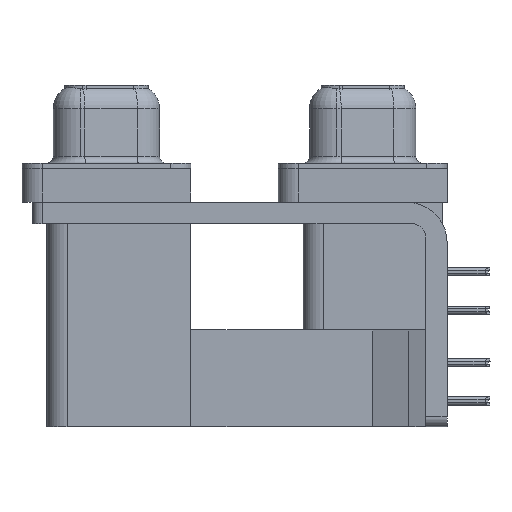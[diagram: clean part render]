
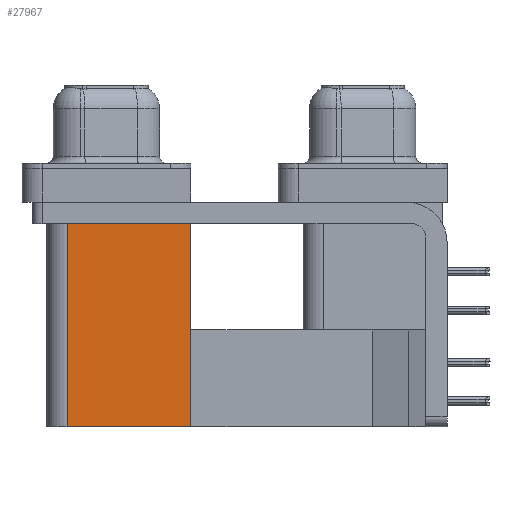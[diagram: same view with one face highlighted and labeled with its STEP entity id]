
A CAD part, left-side view. The second image highlights one B-rep face of the part: STEP entity #27967.
In plain terms, the highlighted planar face has unit normal (-1, 0, 0).
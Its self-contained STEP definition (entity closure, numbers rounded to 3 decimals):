
#82 = CARTESIAN_POINT ( 'NONE',  ( 3.79, 12.775, -19.2 ) ) ;
#305 = LINE ( 'NONE', #22608, #19377 ) ;
#399 = EDGE_CURVE ( 'NONE', #24945, #8483, #24794, .T. ) ;
#3603 = VECTOR ( 'NONE', #15435, 1000. ) ;
#3706 = EDGE_CURVE ( 'NONE', #8483, #28441, #305, .T. ) ;
#7196 = ORIENTED_EDGE ( 'NONE', *, *, #399, .T. ) ;
#8483 = VERTEX_POINT ( 'NONE', #15745 ) ;
#8659 = CARTESIAN_POINT ( 'NONE',  ( 3.79, 12.775, -19.2 ) ) ;
#10541 = CARTESIAN_POINT ( 'NONE',  ( 3.79, 12.775, -19.2 ) ) ;
#11848 = CARTESIAN_POINT ( 'NONE',  ( 3.79, 21.975, -19.2 ) ) ;
#11885 = DIRECTION ( 'NONE',  ( 0., 1., 0. ) ) ;
#13657 = VECTOR ( 'NONE', #25687, 1000. ) ;
#15435 = DIRECTION ( 'NONE',  ( 0., 0., 1. ) ) ;
#15745 = CARTESIAN_POINT ( 'NONE',  ( 3.79, 12.775, -2.5 ) ) ;
#16139 = CARTESIAN_POINT ( 'NONE',  ( 3.79, 21.975, -19.2 ) ) ;
#17267 = EDGE_LOOP ( 'NONE', ( #40820, #27397, #29177, #7196 ) ) ;
#19377 = VECTOR ( 'NONE', #35562, 1000. ) ;
#21002 = CARTESIAN_POINT ( 'NONE',  ( 3.79, 12.775, -19.2 ) ) ;
#22608 = CARTESIAN_POINT ( 'NONE',  ( 3.79, 12.775, -2.5 ) ) ;
#22734 = LINE ( 'NONE', #16139, #13657 ) ;
#23825 = VECTOR ( 'NONE', #11885, 1000. ) ;
#24794 = LINE ( 'NONE', #8659, #3603 ) ;
#24945 = VERTEX_POINT ( 'NONE', #10541 ) ;
#25687 = DIRECTION ( 'NONE',  ( 0., 0., 1. ) ) ;
#26436 = VERTEX_POINT ( 'NONE', #11848 ) ;
#27397 = ORIENTED_EDGE ( 'NONE', *, *, #31486, .F. ) ;
#27967 = ADVANCED_FACE ( 'NONE', ( #28760 ), #32171, .F. ) ;
#28006 = LINE ( 'NONE', #21002, #23825 ) ;
#28441 = VERTEX_POINT ( 'NONE', #35146 ) ;
#28760 = FACE_OUTER_BOUND ( 'NONE', #17267, .T. ) ;
#29177 = ORIENTED_EDGE ( 'NONE', *, *, #30742, .F. ) ;
#30742 = EDGE_CURVE ( 'NONE', #24945, #26436, #28006, .T. ) ;
#31486 = EDGE_CURVE ( 'NONE', #26436, #28441, #22734, .T. ) ;
#32171 = PLANE ( 'NONE',  #36568 ) ;
#34941 = DIRECTION ( 'NONE',  ( 0., 1., 0. ) ) ;
#35146 = CARTESIAN_POINT ( 'NONE',  ( 3.79, 21.975, -2.5 ) ) ;
#35562 = DIRECTION ( 'NONE',  ( 0., 1., 0. ) ) ;
#36568 = AXIS2_PLACEMENT_3D ( 'NONE', #82, #41743, #34941 ) ;
#40820 = ORIENTED_EDGE ( 'NONE', *, *, #3706, .T. ) ;
#41743 = DIRECTION ( 'NONE',  ( 1., 0., 0. ) ) ;
